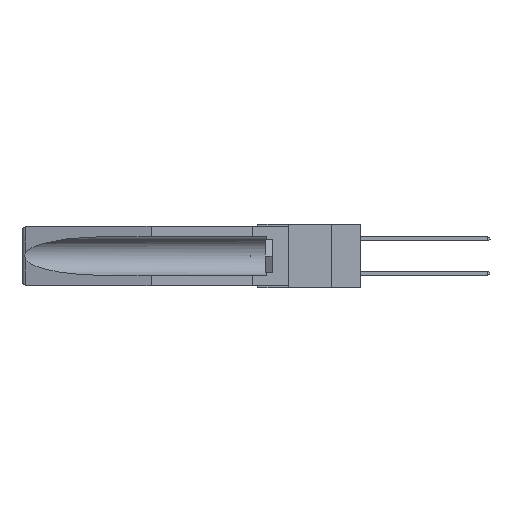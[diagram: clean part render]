
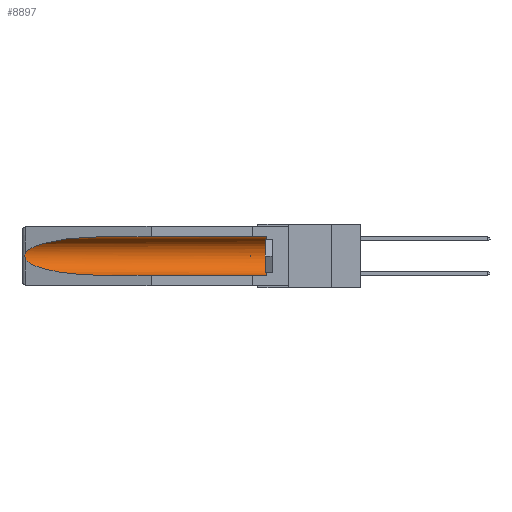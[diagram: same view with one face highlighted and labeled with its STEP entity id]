
A CAD part, left-side view. The second image highlights one B-rep face of the part: STEP entity #8897.
In plain terms, the highlighted cylindrical face has radius 2.857 mm (diameter 5.715 mm), a partial arc.
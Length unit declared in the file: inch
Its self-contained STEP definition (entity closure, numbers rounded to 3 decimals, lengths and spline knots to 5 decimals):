
#1027 = CARTESIAN_POINT ( 'NONE',  ( 0.155, 1.07973, -0.284 ) ) ;
#1032 = CARTESIAN_POINT ( 'NONE',  ( 0.26597, 1.52961, -0.15275 ) ) ;
#3065 = CARTESIAN_POINT ( 'NONE',  ( 0.26537, 1.52718, -0.14972 ) ) ;
#3120 = CARTESIAN_POINT ( 'NONE',  ( 0.26537, 1.52718, -0.14972 ) ) ;
#3494 = VECTOR ( 'NONE', #29004, 39.37008 ) ;
#3956 = VERTEX_POINT ( 'NONE', #1027 ) ;
#4263 = AXIS2_PLACEMENT_3D ( 'NONE', #14782, #22603, #6763 ) ;
#5440 = DIRECTION ( 'NONE',  ( 0., 0., 1. ) ) ;
#5903 = CARTESIAN_POINT ( 'NONE',  ( 0.2673, 1.5327, -0.16383 ) ) ;
#5943 = LINE ( 'NONE', #25060, #10589 ) ;
#6573 = ORIENTED_EDGE ( 'NONE', *, *, #23326, .T. ) ;
#6586 = CARTESIAN_POINT ( 'NONE',  ( 0.155, 1.07973, -0.059 ) ) ;
#6763 = DIRECTION ( 'NONE',  ( 0., 0., 1. ) ) ;
#7937 = CARTESIAN_POINT ( 'NONE',  ( 0.155, -0.30754, -0.1715 ) ) ;
#8612 = CARTESIAN_POINT ( 'NONE',  ( 0.2675, 1.53308, -0.16763 ) ) ;
#8728 = CARTESIAN_POINT ( 'NONE',  ( 0.26654, 1.53092, -0.15636 ) ) ;
#8897 = ADVANCED_FACE ( 'NONE', ( #17586 ), #24425, .F. ) ;
#9629 = EDGE_CURVE ( 'NONE', #27344, #3956, #17702, .T. ) ;
#9918 = CARTESIAN_POINT ( 'NONE',  ( 0.155, -0.30754, -0.059 ) ) ;
#10589 = VECTOR ( 'NONE', #16853, 39.37008 ) ;
#10826 = EDGE_CURVE ( 'NONE', #16869, #13192, #27656, .T. ) ;
#11306 = ORIENTED_EDGE ( 'NONE', *, *, #10826, .T. ) ;
#11316 = CARTESIAN_POINT ( 'NONE',  ( 0.26655, 1.53094, -0.18657 ) ) ;
#11362 = CARTESIAN_POINT ( 'NONE',  ( 0.155, 0.126, -0.059 ) ) ;
#11578 = EDGE_LOOP ( 'NONE', ( #29908, #6573, #12496, #13272, #16999, #11306 ) ) ;
#12496 = ORIENTED_EDGE ( 'NONE', *, *, #9629, .T. ) ;
#12734 = EDGE_CURVE ( 'NONE', #32283, #16869, #31344, .T. ) ;
#13192 = VERTEX_POINT ( 'NONE', #6586 ) ;
#13272 = ORIENTED_EDGE ( 'NONE', *, *, #31575, .F. ) ;
#14782 = CARTESIAN_POINT ( 'NONE',  ( 0.155, 0.126, -0.1715 ) ) ;
#15336 = CARTESIAN_POINT ( 'NONE',  ( 0.26597, 1.5296, -0.19026 ) ) ;
#15395 = VERTEX_POINT ( 'NONE', #3120 ) ;
#15746 = CARTESIAN_POINT ( 'NONE',  ( 0.26537, 1.52718, -0.19328 ) ) ;
#16853 = DIRECTION ( 'NONE',  ( 0., 1., 0. ) ) ;
#16869 = VERTEX_POINT ( 'NONE', #11362 ) ;
#16999 = ORIENTED_EDGE ( 'NONE', *, *, #12734, .T. ) ;
#17586 = FACE_OUTER_BOUND ( 'NONE', #11578, .T. ) ;
#17702 =( BOUNDED_CURVE ( )  B_SPLINE_CURVE ( 3, ( #15746, #34734, #18447, #18109 ),
 .UNSPECIFIED., .F., .T. ) 
 B_SPLINE_CURVE_WITH_KNOTS ( ( 4, 4 ),
 ( 0.1948, 1.5708 ),
 .UNSPECIFIED. ) 
 CURVE ( )  GEOMETRIC_REPRESENTATION_ITEM ( )  RATIONAL_B_SPLINE_CURVE ( ( 1., 0.848, 0.848, 1. ) ) 
 REPRESENTATION_ITEM ( '' )  );
#18109 = CARTESIAN_POINT ( 'NONE',  ( 0.155, 1.07973, -0.284 ) ) ;
#18447 = CARTESIAN_POINT ( 'NONE',  ( 0.21114, 1.30732, -0.284 ) ) ;
#20143 = EDGE_CURVE ( 'NONE', #13192, #15395, #31963, .T. ) ;
#22464 = CARTESIAN_POINT ( 'NONE',  ( 0.155, 1.07973, -0.059 ) ) ;
#22603 = DIRECTION ( 'NONE',  ( 0., -1., 0. ) ) ;
#23326 = EDGE_CURVE ( 'NONE', #15395, #27344, #24051, .T. ) ;
#23947 = CARTESIAN_POINT ( 'NONE',  ( 0.155, 0.126, -0.284 ) ) ;
#24051 = B_SPLINE_CURVE_WITH_KNOTS ( 'NONE', 3,
 ( #27934, #1032, #8728, #5903, #8612, #27579, #27690, #11316, #15336, #29026 ),
 .UNSPECIFIED., .F., .F.,
 ( 4, 2, 2, 2, 4 ),
 ( 0., 0.00029, 0.00058, 0.00087, 0.00117 ),
 .UNSPECIFIED. ) ;
#24425 = CYLINDRICAL_SURFACE ( 'NONE', #24579, 0.1125 ) ;
#24579 = AXIS2_PLACEMENT_3D ( 'NONE', #7937, #29530, #5440 ) ;
#24967 = CARTESIAN_POINT ( 'NONE',  ( 0.21114, 1.30732, -0.059 ) ) ;
#25060 = CARTESIAN_POINT ( 'NONE',  ( 0.155, -0.30754, -0.284 ) ) ;
#27344 = VERTEX_POINT ( 'NONE', #27843 ) ;
#27477 = CARTESIAN_POINT ( 'NONE',  ( 0.25451, 1.48313, -0.09465 ) ) ;
#27579 = CARTESIAN_POINT ( 'NONE',  ( 0.2675, 1.53308, -0.17534 ) ) ;
#27656 = LINE ( 'NONE', #9918, #3494 ) ;
#27690 = CARTESIAN_POINT ( 'NONE',  ( 0.2673, 1.53269, -0.17917 ) ) ;
#27843 = CARTESIAN_POINT ( 'NONE',  ( 0.26537, 1.52718, -0.19328 ) ) ;
#27934 = CARTESIAN_POINT ( 'NONE',  ( 0.26537, 1.52718, -0.14972 ) ) ;
#29004 = DIRECTION ( 'NONE',  ( 0., 1., 0. ) ) ;
#29026 = CARTESIAN_POINT ( 'NONE',  ( 0.26537, 1.52718, -0.19328 ) ) ;
#29530 = DIRECTION ( 'NONE',  ( 0., 1., 0. ) ) ;
#29908 = ORIENTED_EDGE ( 'NONE', *, *, #20143, .T. ) ;
#31344 = CIRCLE ( 'NONE', #4263, 0.1125 ) ;
#31575 = EDGE_CURVE ( 'NONE', #32283, #3956, #5943, .T. ) ;
#31963 =( BOUNDED_CURVE ( )  B_SPLINE_CURVE ( 3, ( #22464, #24967, #27477, #3065 ),
 .UNSPECIFIED., .F., .T. ) 
 B_SPLINE_CURVE_WITH_KNOTS ( ( 4, 4 ),
 ( 4.71239, 6.08839 ),
 .UNSPECIFIED. ) 
 CURVE ( )  GEOMETRIC_REPRESENTATION_ITEM ( )  RATIONAL_B_SPLINE_CURVE ( ( 1., 0.848, 0.848, 1. ) ) 
 REPRESENTATION_ITEM ( '' )  );
#32283 = VERTEX_POINT ( 'NONE', #23947 ) ;
#34734 = CARTESIAN_POINT ( 'NONE',  ( 0.25451, 1.48313, -0.24835 ) ) ;
